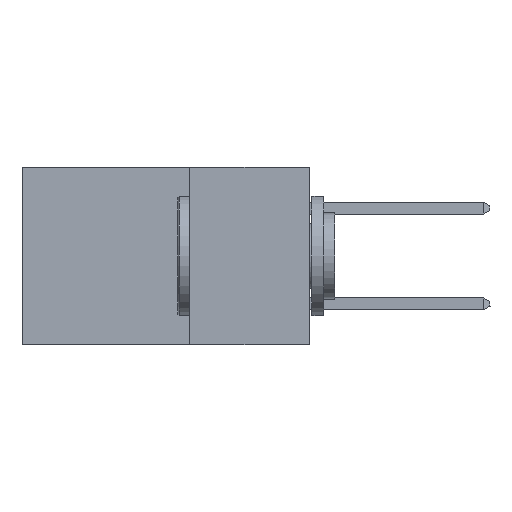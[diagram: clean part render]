
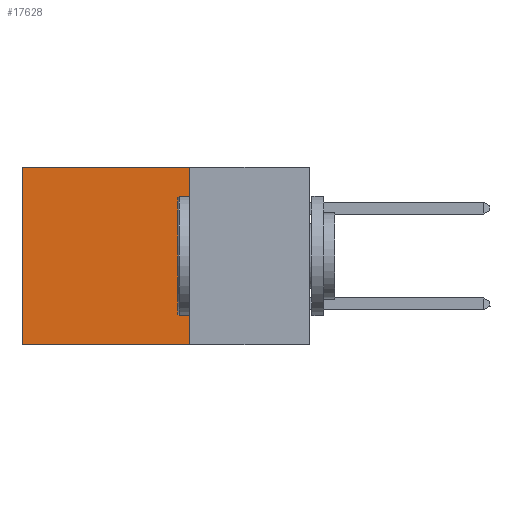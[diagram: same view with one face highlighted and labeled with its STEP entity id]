
A CAD part, left-side view. The second image highlights one B-rep face of the part: STEP entity #17628.
In plain terms, the highlighted planar face has unit normal (-1, 0, 0).
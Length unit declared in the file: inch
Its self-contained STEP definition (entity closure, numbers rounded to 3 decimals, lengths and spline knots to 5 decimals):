
#218 = ORIENTED_EDGE ( 'NONE', *, *, #5562, .T. ) ;
#1304 = CARTESIAN_POINT ( 'NONE',  ( 0.2875, 0.25, 0. ) ) ;
#2500 = EDGE_CURVE ( 'NONE', #27040, #28738, #13702, .T. ) ;
#2648 = ORIENTED_EDGE ( 'NONE', *, *, #2500, .T. ) ;
#3230 = FACE_OUTER_BOUND ( 'NONE', #12022, .T. ) ;
#5562 = EDGE_CURVE ( 'NONE', #20700, #27040, #11921, .T. ) ;
#5658 = VERTEX_POINT ( 'NONE', #17023 ) ;
#5876 = PLANE ( 'NONE',  #13656 ) ;
#7125 = VECTOR ( 'NONE', #25323, 39.37008 ) ;
#7872 = CARTESIAN_POINT ( 'NONE',  ( 0.2875, 0.25, 0. ) ) ;
#11921 = LINE ( 'NONE', #1304, #12300 ) ;
#12022 = EDGE_LOOP ( 'NONE', ( #2648, #24481, #18989, #218 ) ) ;
#12300 = VECTOR ( 'NONE', #23733, 39.37008 ) ;
#13656 = AXIS2_PLACEMENT_3D ( 'NONE', #21138, #15849, #23632 ) ;
#13702 = LINE ( 'NONE', #27403, #7125 ) ;
#14507 = DIRECTION ( 'NONE',  ( 0., 1., 0. ) ) ;
#15849 = DIRECTION ( 'NONE',  ( 1., 0., 0. ) ) ;
#17023 = CARTESIAN_POINT ( 'NONE',  ( 0.2875, 0.25, -0.37 ) ) ;
#17628 = ADVANCED_FACE ( 'NONE', ( #3230 ), #5876, .F. ) ;
#17861 = VECTOR ( 'NONE', #14507, 39.37008 ) ;
#18166 = DIRECTION ( 'NONE',  ( 0., 0., -1. ) ) ;
#18989 = ORIENTED_EDGE ( 'NONE', *, *, #29563, .F. ) ;
#20700 = VERTEX_POINT ( 'NONE', #26144 ) ;
#21138 = CARTESIAN_POINT ( 'NONE',  ( 0.2875, 0.25, 0. ) ) ;
#21957 = EDGE_CURVE ( 'NONE', #5658, #28738, #25994, .T. ) ;
#23408 = VECTOR ( 'NONE', #18166, 39.37008 ) ;
#23632 = DIRECTION ( 'NONE',  ( 0., 0., -1. ) ) ;
#23733 = DIRECTION ( 'NONE',  ( 0., 1., 0. ) ) ;
#23925 = CARTESIAN_POINT ( 'NONE',  ( 0.2875, 0.6, -0.37 ) ) ;
#24481 = ORIENTED_EDGE ( 'NONE', *, *, #21957, .F. ) ;
#25323 = DIRECTION ( 'NONE',  ( 0., 0., -1. ) ) ;
#25994 = LINE ( 'NONE', #29368, #17861 ) ;
#26144 = CARTESIAN_POINT ( 'NONE',  ( 0.2875, 0.25, 0. ) ) ;
#27040 = VERTEX_POINT ( 'NONE', #30423 ) ;
#27403 = CARTESIAN_POINT ( 'NONE',  ( 0.2875, 0.6, 0. ) ) ;
#28072 = LINE ( 'NONE', #7872, #23408 ) ;
#28738 = VERTEX_POINT ( 'NONE', #23925 ) ;
#29368 = CARTESIAN_POINT ( 'NONE',  ( 0.2875, 0.25, -0.37 ) ) ;
#29563 = EDGE_CURVE ( 'NONE', #20700, #5658, #28072, .T. ) ;
#30423 = CARTESIAN_POINT ( 'NONE',  ( 0.2875, 0.6, 0. ) ) ;
